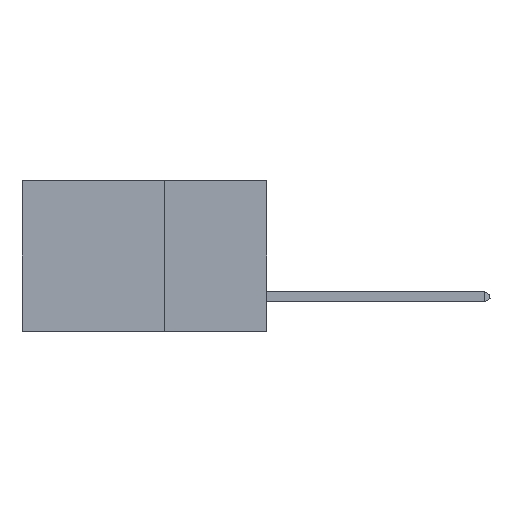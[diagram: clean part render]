
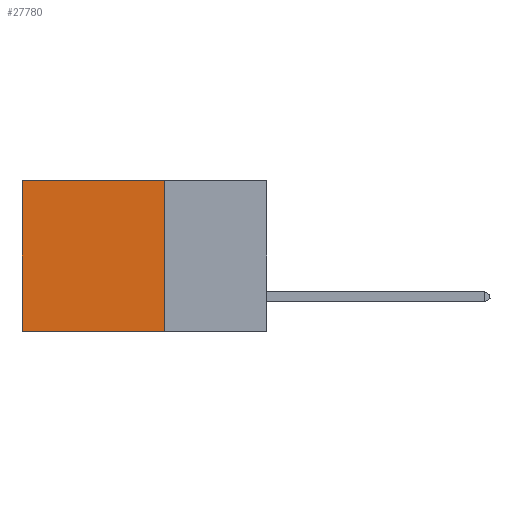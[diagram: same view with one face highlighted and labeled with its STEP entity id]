
A CAD part, left-side view. The second image highlights one B-rep face of the part: STEP entity #27780.
In plain terms, the highlighted planar face has unit normal (-1, 0, 0).
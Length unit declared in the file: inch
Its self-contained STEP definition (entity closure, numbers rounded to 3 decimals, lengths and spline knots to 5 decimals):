
#34 = CARTESIAN_POINT ( 'NONE',  ( 0.2875, 0.25, -0.37 ) ) ;
#4402 = CARTESIAN_POINT ( 'NONE',  ( 0.2875, 0.6, 0. ) ) ;
#4761 = VERTEX_POINT ( 'NONE', #20440 ) ;
#4766 = AXIS2_PLACEMENT_3D ( 'NONE', #18089, #18185, #13949 ) ;
#4816 = EDGE_LOOP ( 'NONE', ( #10647, #17025, #12594, #9672 ) ) ;
#7089 = EDGE_CURVE ( 'NONE', #19719, #27598, #10238, .T. ) ;
#7134 = LINE ( 'NONE', #21753, #16257 ) ;
#7152 = CARTESIAN_POINT ( 'NONE',  ( 0.2875, 0.25, -0.37 ) ) ;
#7439 = PLANE ( 'NONE',  #4766 ) ;
#8432 = CARTESIAN_POINT ( 'NONE',  ( 0.2875, 0.25, 0. ) ) ;
#8915 = VECTOR ( 'NONE', #25004, 39.37008 ) ;
#9052 = FACE_OUTER_BOUND ( 'NONE', #4816, .T. ) ;
#9672 = ORIENTED_EDGE ( 'NONE', *, *, #25775, .T. ) ;
#10238 = LINE ( 'NONE', #4402, #8915 ) ;
#10647 = ORIENTED_EDGE ( 'NONE', *, *, #7089, .T. ) ;
#10968 = VECTOR ( 'NONE', #25369, 39.37008 ) ;
#11293 = DIRECTION ( 'NONE',  ( 0., 1., 0. ) ) ;
#12594 = ORIENTED_EDGE ( 'NONE', *, *, #23796, .F. ) ;
#13079 = DIRECTION ( 'NONE',  ( 0., 1., 0. ) ) ;
#13654 = VERTEX_POINT ( 'NONE', #34 ) ;
#13949 = DIRECTION ( 'NONE',  ( 0., 0., -1. ) ) ;
#16257 = VECTOR ( 'NONE', #13079, 39.37008 ) ;
#16631 = LINE ( 'NONE', #7152, #24378 ) ;
#17025 = ORIENTED_EDGE ( 'NONE', *, *, #18201, .F. ) ;
#18089 = CARTESIAN_POINT ( 'NONE',  ( 0.2875, 0.25, 0. ) ) ;
#18185 = DIRECTION ( 'NONE',  ( 1., 0., 0. ) ) ;
#18201 = EDGE_CURVE ( 'NONE', #13654, #27598, #16631, .T. ) ;
#19719 = VERTEX_POINT ( 'NONE', #23187 ) ;
#20440 = CARTESIAN_POINT ( 'NONE',  ( 0.2875, 0.25, 0. ) ) ;
#21753 = CARTESIAN_POINT ( 'NONE',  ( 0.2875, 0.25, 0. ) ) ;
#23105 = LINE ( 'NONE', #8432, #10968 ) ;
#23187 = CARTESIAN_POINT ( 'NONE',  ( 0.2875, 0.6, 0. ) ) ;
#23796 = EDGE_CURVE ( 'NONE', #4761, #13654, #23105, .T. ) ;
#24289 = CARTESIAN_POINT ( 'NONE',  ( 0.2875, 0.6, -0.37 ) ) ;
#24378 = VECTOR ( 'NONE', #11293, 39.37008 ) ;
#25004 = DIRECTION ( 'NONE',  ( 0., 0., -1. ) ) ;
#25369 = DIRECTION ( 'NONE',  ( 0., 0., -1. ) ) ;
#25775 = EDGE_CURVE ( 'NONE', #4761, #19719, #7134, .T. ) ;
#27598 = VERTEX_POINT ( 'NONE', #24289 ) ;
#27780 = ADVANCED_FACE ( 'NONE', ( #9052 ), #7439, .F. ) ;
